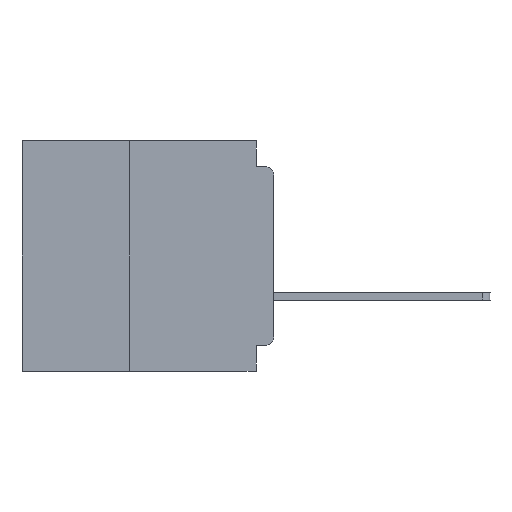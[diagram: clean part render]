
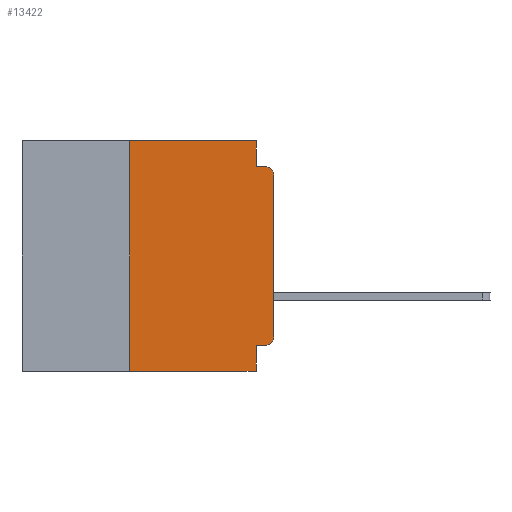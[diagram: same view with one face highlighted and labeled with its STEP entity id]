
A CAD part, left-side view. The second image highlights one B-rep face of the part: STEP entity #13422.
In plain terms, the highlighted planar face has unit normal (-1, 0, 0).
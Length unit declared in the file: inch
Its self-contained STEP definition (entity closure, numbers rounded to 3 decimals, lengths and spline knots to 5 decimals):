
#89 = EDGE_CURVE ( 'NONE', #12095, #22573, #4191, .T. ) ;
#198 = LINE ( 'NONE', #38817, #23093 ) ;
#341 = ORIENTED_EDGE ( 'NONE', *, *, #24594, .F. ) ;
#911 = ORIENTED_EDGE ( 'NONE', *, *, #52754, .F. ) ;
#1190 = CARTESIAN_POINT ( 'NONE',  ( 0., 0., -0.045 ) ) ;
#1345 = CARTESIAN_POINT ( 'NONE',  ( 0., 0.031, -0.045 ) ) ;
#1623 = CARTESIAN_POINT ( 'NONE',  ( 0., 0., -0.06 ) ) ;
#1796 = LINE ( 'NONE', #1190, #24693 ) ;
#2486 = DIRECTION ( 'NONE',  ( 0., 1., 0. ) ) ;
#2556 = DIRECTION ( 'NONE',  ( 0., -1., 0. ) ) ;
#2746 = VERTEX_POINT ( 'NONE', #54212 ) ;
#3036 = DIRECTION ( 'NONE',  ( 1., 0., 0. ) ) ;
#4191 = LINE ( 'NONE', #27213, #27022 ) ;
#4689 = CARTESIAN_POINT ( 'NONE',  ( 0., 0., -0.34 ) ) ;
#4765 = CARTESIAN_POINT ( 'NONE',  ( 0., 0.015, -0.06 ) ) ;
#5975 = AXIS2_PLACEMENT_3D ( 'NONE', #4765, #36597, #9378 ) ;
#6573 = VECTOR ( 'NONE', #43821, 39.37008 ) ;
#7461 = PLANE ( 'NONE',  #20400 ) ;
#7465 = CARTESIAN_POINT ( 'NONE',  ( 0., 0.25, 0. ) ) ;
#8396 = FACE_OUTER_BOUND ( 'NONE', #31344, .T. ) ;
#9378 = DIRECTION ( 'NONE',  ( 0., 0., -1. ) ) ;
#9936 = LINE ( 'NONE', #35676, #46970 ) ;
#10381 = LINE ( 'NONE', #57421, #33115 ) ;
#10530 = ORIENTED_EDGE ( 'NONE', *, *, #41835, .T. ) ;
#10620 = DIRECTION ( 'NONE',  ( 0., -1., 0. ) ) ;
#11239 = DIRECTION ( 'NONE',  ( -1., 0., 0. ) ) ;
#12095 = VERTEX_POINT ( 'NONE', #38027 ) ;
#12389 = VERTEX_POINT ( 'NONE', #17770 ) ;
#13241 = VERTEX_POINT ( 'NONE', #1623 ) ;
#13422 = ADVANCED_FACE ( 'NONE', ( #8396 ), #7461, .F. ) ;
#15069 = CIRCLE ( 'NONE', #53581, 0.015 ) ;
#16345 = ORIENTED_EDGE ( 'NONE', *, *, #20505, .F. ) ;
#17625 = ORIENTED_EDGE ( 'NONE', *, *, #34774, .F. ) ;
#17770 = CARTESIAN_POINT ( 'NONE',  ( 0., 0.015, -0.045 ) ) ;
#18617 = CIRCLE ( 'NONE', #5975, 0.015 ) ;
#18785 = LINE ( 'NONE', #34458, #42866 ) ;
#19361 = EDGE_CURVE ( 'NONE', #2746, #46695, #15069, .T. ) ;
#20400 = AXIS2_PLACEMENT_3D ( 'NONE', #52784, #3036, #34912 ) ;
#20505 = EDGE_CURVE ( 'NONE', #23382, #12095, #9936, .T. ) ;
#20748 = DIRECTION ( 'NONE',  ( 0., 0., -1. ) ) ;
#22573 = VERTEX_POINT ( 'NONE', #1345 ) ;
#23093 = VECTOR ( 'NONE', #20748, 39.37008 ) ;
#23382 = VERTEX_POINT ( 'NONE', #7465 ) ;
#24594 = EDGE_CURVE ( 'NONE', #2746, #48507, #56390, .T. ) ;
#24693 = VECTOR ( 'NONE', #10620, 39.37008 ) ;
#25675 = DIRECTION ( 'NONE',  ( 0., 0., 1. ) ) ;
#26781 = DIRECTION ( 'NONE',  ( 0., -1., 0. ) ) ;
#26902 = DIRECTION ( 'NONE',  ( 0., 0., -1. ) ) ;
#27022 = VECTOR ( 'NONE', #26902, 39.37008 ) ;
#27213 = CARTESIAN_POINT ( 'NONE',  ( 0., 0.031, 0. ) ) ;
#27637 = ORIENTED_EDGE ( 'NONE', *, *, #19361, .T. ) ;
#31229 = VERTEX_POINT ( 'NONE', #36374 ) ;
#31344 = EDGE_LOOP ( 'NONE', ( #35874, #10530, #911, #34461, #16345, #33770, #38105, #17625, #341, #27637 ) ) ;
#32000 = VERTEX_POINT ( 'NONE', #40138 ) ;
#32194 = LINE ( 'NONE', #39296, #6573 ) ;
#33115 = VECTOR ( 'NONE', #25675, 39.37008 ) ;
#33770 = ORIENTED_EDGE ( 'NONE', *, *, #58576, .F. ) ;
#34385 = CARTESIAN_POINT ( 'NONE',  ( 0., 0., -0.355 ) ) ;
#34458 = CARTESIAN_POINT ( 'NONE',  ( 0., 0.437, -0.4 ) ) ;
#34461 = ORIENTED_EDGE ( 'NONE', *, *, #89, .F. ) ;
#34774 = EDGE_CURVE ( 'NONE', #48507, #31229, #198, .T. ) ;
#34912 = DIRECTION ( 'NONE',  ( 0., 0., -1. ) ) ;
#35676 = CARTESIAN_POINT ( 'NONE',  ( 0., 0.437, 0. ) ) ;
#35874 = ORIENTED_EDGE ( 'NONE', *, *, #40940, .T. ) ;
#36374 = CARTESIAN_POINT ( 'NONE',  ( 0., 0.031, -0.4 ) ) ;
#36597 = DIRECTION ( 'NONE',  ( -1., 0., 0. ) ) ;
#38027 = CARTESIAN_POINT ( 'NONE',  ( 0., 0.031, 0. ) ) ;
#38105 = ORIENTED_EDGE ( 'NONE', *, *, #43498, .T. ) ;
#38473 = CARTESIAN_POINT ( 'NONE',  ( 0., 0.015, -0.34 ) ) ;
#38817 = CARTESIAN_POINT ( 'NONE',  ( 0., 0.031, -0.4 ) ) ;
#39296 = CARTESIAN_POINT ( 'NONE',  ( 0., 0., 0. ) ) ;
#40138 = CARTESIAN_POINT ( 'NONE',  ( 0., 0.25, -0.4 ) ) ;
#40940 = EDGE_CURVE ( 'NONE', #46695, #13241, #32194, .T. ) ;
#41835 = EDGE_CURVE ( 'NONE', #13241, #12389, #18617, .T. ) ;
#42866 = VECTOR ( 'NONE', #2556, 39.37008 ) ;
#43002 = DIRECTION ( 'NONE',  ( 0., 0., -1. ) ) ;
#43498 = EDGE_CURVE ( 'NONE', #32000, #31229, #18785, .T. ) ;
#43821 = DIRECTION ( 'NONE',  ( 0., 0., 1. ) ) ;
#45728 = VECTOR ( 'NONE', #2486, 39.37008 ) ;
#46695 = VERTEX_POINT ( 'NONE', #4689 ) ;
#46970 = VECTOR ( 'NONE', #26781, 39.37008 ) ;
#48507 = VERTEX_POINT ( 'NONE', #49844 ) ;
#49844 = CARTESIAN_POINT ( 'NONE',  ( 0., 0.031, -0.355 ) ) ;
#52754 = EDGE_CURVE ( 'NONE', #22573, #12389, #1796, .T. ) ;
#52784 = CARTESIAN_POINT ( 'NONE',  ( 0., 0.437, 0. ) ) ;
#53581 = AXIS2_PLACEMENT_3D ( 'NONE', #38473, #11239, #43002 ) ;
#54212 = CARTESIAN_POINT ( 'NONE',  ( 0., 0.015, -0.355 ) ) ;
#56390 = LINE ( 'NONE', #34385, #45728 ) ;
#57421 = CARTESIAN_POINT ( 'NONE',  ( 0., 0.25, -0.4 ) ) ;
#58576 = EDGE_CURVE ( 'NONE', #32000, #23382, #10381, .T. ) ;
